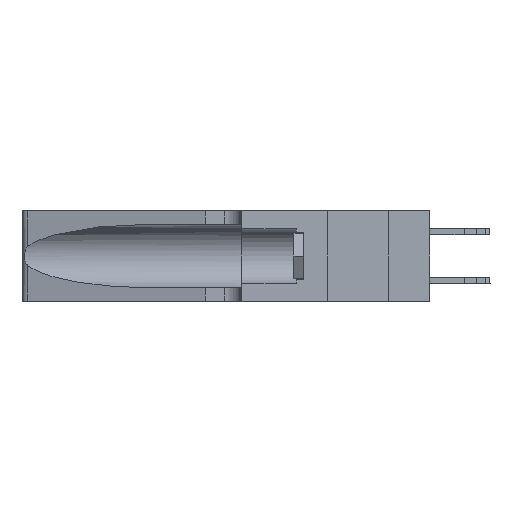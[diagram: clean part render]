
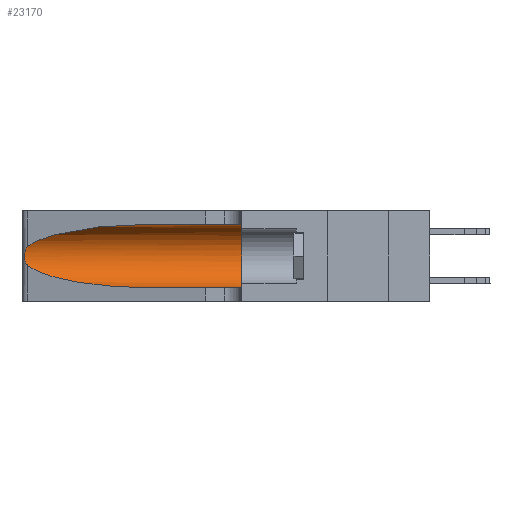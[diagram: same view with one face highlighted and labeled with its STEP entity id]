
A CAD part, left-side view. The second image highlights one B-rep face of the part: STEP entity #23170.
In plain terms, the highlighted cylindrical face has radius 3.308 mm (diameter 6.617 mm), a partial arc.
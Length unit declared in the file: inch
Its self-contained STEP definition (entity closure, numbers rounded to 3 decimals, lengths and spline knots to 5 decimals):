
#655 = ORIENTED_EDGE ( 'NONE', *, *, #11316, .T. ) ;
#1292 = CARTESIAN_POINT ( 'NONE',  ( 0.25487, 1.22718, 0.14631 ) ) ;
#1891 = VERTEX_POINT ( 'NONE', #3818 ) ;
#2794 = VERTEX_POINT ( 'NONE', #10171 ) ;
#3718 = CARTESIAN_POINT ( 'NONE',  ( 0.25555, 1.22994, 0.2215 ) ) ;
#3818 = CARTESIAN_POINT ( 'NONE',  ( 0.1305, 0.35, 0.05475 ) ) ;
#4218 = CARTESIAN_POINT ( 'NONE',  ( 0.26017, 1.23833, 0.17102 ) ) ;
#4961 = DIRECTION ( 'NONE',  ( 0., 1., 0. ) ) ;
#6007 = ORIENTED_EDGE ( 'NONE', *, *, #18982, .F. ) ;
#6170 = EDGE_LOOP ( 'NONE', ( #8704, #10749, #15192, #655, #6007, #26897 ) ) ;
#6370 = CARTESIAN_POINT ( 'NONE',  ( 0.25639, 1.23186, 0.15144 ) ) ;
#6436 = CARTESIAN_POINT ( 'NONE',  ( 0.2373, 1.15595, 0.28018 ) ) ;
#6743 = DIRECTION ( 'NONE',  ( 0., -1., 0. ) ) ;
#7460 = VECTOR ( 'NONE', #24516, 39.37008 ) ;
#7514 = EDGE_CURVE ( 'NONE', #18495, #28508, #30320, .T. ) ;
#7688 = CARTESIAN_POINT ( 'NONE',  ( 0.1305, 1.61858, 0.185 ) ) ;
#8138 = AXIS2_PLACEMENT_3D ( 'NONE', #7688, #23093, #26021 ) ;
#8704 = ORIENTED_EDGE ( 'NONE', *, *, #24185, .T. ) ;
#9435 = CARTESIAN_POINT ( 'NONE',  ( 0.1305, 0.72297, 0.05475 ) ) ;
#9449 = LINE ( 'NONE', #24753, #7460 ) ;
#10171 = CARTESIAN_POINT ( 'NONE',  ( 0.1305, 0.35, 0.31525 ) ) ;
#10749 = ORIENTED_EDGE ( 'NONE', *, *, #7514, .T. ) ;
#10868 = EDGE_CURVE ( 'NONE', #25111, #2794, #9449, .T. ) ;
#11177 = FACE_OUTER_BOUND ( 'NONE', #6170, .T. ) ;
#11316 = EDGE_CURVE ( 'NONE', #11810, #1891, #23181, .T. ) ;
#11624 = CARTESIAN_POINT ( 'NONE',  ( 0.25487, 1.22718, 0.22369 ) ) ;
#11735 = CARTESIAN_POINT ( 'NONE',  ( 0.26018, 1.23835, 0.19895 ) ) ;
#11810 = VERTEX_POINT ( 'NONE', #25325 ) ;
#11979 = CARTESIAN_POINT ( 'NONE',  ( 0.25639, 1.23184, 0.21858 ) ) ;
#14340 = CARTESIAN_POINT ( 'NONE',  ( 0.26075, 1.23896, 0.178 ) ) ;
#15192 = ORIENTED_EDGE ( 'NONE', *, *, #32133, .T. ) ;
#16287 = CIRCLE ( 'NONE', #19705, 0.13025 ) ;
#16584 = CARTESIAN_POINT ( 'NONE',  ( 0.25487, 1.22718, 0.22369 ) ) ;
#16985 = CARTESIAN_POINT ( 'NONE',  ( 0.25555, 1.22993, 0.14849 ) ) ;
#17234 = CARTESIAN_POINT ( 'NONE',  ( 0.25856, 1.23593, 0.16098 ) ) ;
#17621 = CARTESIAN_POINT ( 'NONE',  ( 0.1305, 0.72297, 0.31525 ) ) ;
#18495 = VERTEX_POINT ( 'NONE', #27152 ) ;
#18543 = CYLINDRICAL_SURFACE ( 'NONE', #8138, 0.13025 ) ;
#18982 = EDGE_CURVE ( 'NONE', #2794, #1891, #16287, .T. ) ;
#19008 = CARTESIAN_POINT ( 'NONE',  ( 0.18966, 0.96281, 0.31525 ) ) ;
#19705 = AXIS2_PLACEMENT_3D ( 'NONE', #28337, #4961, #23219 ) ;
#19813 = CARTESIAN_POINT ( 'NONE',  ( 0.25487, 1.22718, 0.14631 ) ) ;
#19880 = VECTOR ( 'NONE', #6743, 39.37008 ) ;
#20048 = CARTESIAN_POINT ( 'NONE',  ( 0.2373, 1.15595, 0.08982 ) ) ;
#22274 = CARTESIAN_POINT ( 'NONE',  ( 0.25789, 1.23486, 0.15765 ) ) ;
#23093 = DIRECTION ( 'NONE',  ( 0., -1., 0. ) ) ;
#23170 = ADVANCED_FACE ( 'NONE', ( #11177 ), #18543, .F. ) ;
#23181 = LINE ( 'NONE', #29884, #19880 ) ;
#23219 = DIRECTION ( 'NONE',  ( 0., 0., 1. ) ) ;
#23921 =( BOUNDED_CURVE ( )  B_SPLINE_CURVE ( 3, ( #29063, #19008, #6436, #16584 ),
 .UNSPECIFIED., .F., .F. ) 
 B_SPLINE_CURVE_WITH_KNOTS ( ( 4, 4 ),
 ( 1.5708, 2.84003 ),
 .UNSPECIFIED. ) 
 CURVE ( )  GEOMETRIC_REPRESENTATION_ITEM ( )  RATIONAL_B_SPLINE_CURVE ( ( 1., 0.87, 0.87, 1. ) ) 
 REPRESENTATION_ITEM ( '' )  );
#24185 = EDGE_CURVE ( 'NONE', #25111, #18495, #23921, .T. ) ;
#24516 = DIRECTION ( 'NONE',  ( 0., -1., 0. ) ) ;
#24692 = CARTESIAN_POINT ( 'NONE',  ( 0.18966, 0.96281, 0.05475 ) ) ;
#24753 = CARTESIAN_POINT ( 'NONE',  ( 0.1305, 1.61858, 0.31525 ) ) ;
#25111 = VERTEX_POINT ( 'NONE', #17621 ) ;
#25325 = CARTESIAN_POINT ( 'NONE',  ( 0.1305, 0.72297, 0.05475 ) ) ;
#26021 = DIRECTION ( 'NONE',  ( 0., 0., -1. ) ) ;
#26897 = ORIENTED_EDGE ( 'NONE', *, *, #10868, .F. ) ;
#27152 = CARTESIAN_POINT ( 'NONE',  ( 0.25487, 1.22718, 0.22369 ) ) ;
#27357 = CARTESIAN_POINT ( 'NONE',  ( 0.25854, 1.2359, 0.20912 ) ) ;
#28337 = CARTESIAN_POINT ( 'NONE',  ( 0.1305, 0.35, 0.185 ) ) ;
#28508 = VERTEX_POINT ( 'NONE', #32963 ) ;
#29063 = CARTESIAN_POINT ( 'NONE',  ( 0.1305, 0.72297, 0.31525 ) ) ;
#29884 = CARTESIAN_POINT ( 'NONE',  ( 0.1305, 1.61858, 0.05475 ) ) ;
#30022 = CARTESIAN_POINT ( 'NONE',  ( 0.26075, 1.23896, 0.19203 ) ) ;
#30320 = B_SPLINE_CURVE_WITH_KNOTS ( 'NONE', 3,
 ( #11624, #3718, #11979, #32675, #27357, #11735, #30022, #14340, #4218, #17234, #22274, #6370, #16985, #1292 ),
 .UNSPECIFIED., .F., .F.,
 ( 4, 2, 2, 2, 2, 2, 4 ),
 ( 0., 0.00027, 0.00053, 0.00107, 0.0016, 0.00187, 0.00214 ),
 .UNSPECIFIED. ) ;
#31396 =( BOUNDED_CURVE ( )  B_SPLINE_CURVE ( 3, ( #19813, #20048, #24692, #9435 ),
 .UNSPECIFIED., .F., .T. ) 
 B_SPLINE_CURVE_WITH_KNOTS ( ( 4, 4 ),
 ( 3.44316, 4.71239 ),
 .UNSPECIFIED. ) 
 CURVE ( )  GEOMETRIC_REPRESENTATION_ITEM ( )  RATIONAL_B_SPLINE_CURVE ( ( 1., 0.87, 0.87, 1. ) ) 
 REPRESENTATION_ITEM ( '' )  );
#32133 = EDGE_CURVE ( 'NONE', #28508, #11810, #31396, .T. ) ;
#32675 = CARTESIAN_POINT ( 'NONE',  ( 0.25787, 1.23484, 0.2124 ) ) ;
#32963 = CARTESIAN_POINT ( 'NONE',  ( 0.25487, 1.22718, 0.14631 ) ) ;
